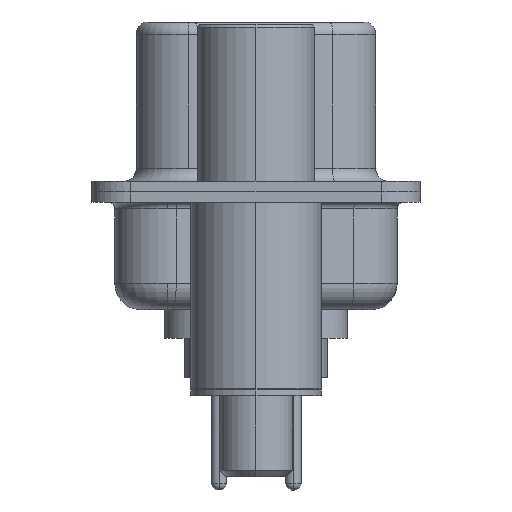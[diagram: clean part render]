
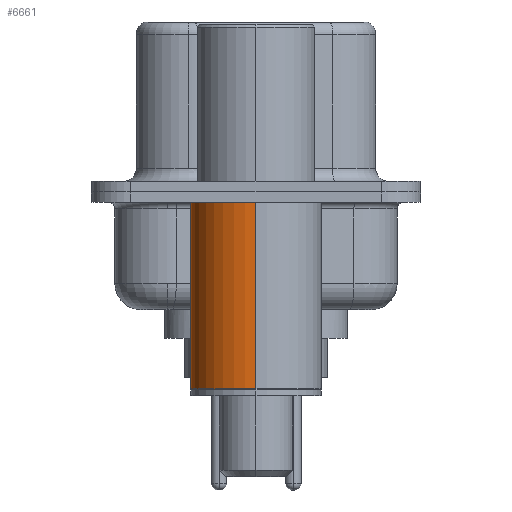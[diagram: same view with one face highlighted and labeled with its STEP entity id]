
A CAD part, left-side view. The second image highlights one B-rep face of the part: STEP entity #6661.
In plain terms, the highlighted cylindrical face has radius 2.5 mm (diameter 5 mm), a partial arc.
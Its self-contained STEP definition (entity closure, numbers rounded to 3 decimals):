
#350 = DIRECTION ( 'NONE',  ( 1., 0., 0. ) ) ;
#1232 = VERTEX_POINT ( 'NONE', #16352 ) ;
#1234 = VERTEX_POINT ( 'NONE', #18870 ) ;
#1271 = DIRECTION ( 'NONE',  ( 1., 0., 0. ) ) ;
#1822 = ORIENTED_EDGE ( 'NONE', *, *, #8953, .T. ) ;
#3179 = AXIS2_PLACEMENT_3D ( 'NONE', #19031, #9683, #350 ) ;
#3250 = CARTESIAN_POINT ( 'NONE',  ( 2.5, 0., -7.525 ) ) ;
#3787 = EDGE_CURVE ( 'NONE', #10739, #1232, #9928, .T. ) ;
#4009 = VECTOR ( 'NONE', #15874, 1000. ) ;
#4331 = DIRECTION ( 'NONE',  ( 1., 0., 0. ) ) ;
#5615 = AXIS2_PLACEMENT_3D ( 'NONE', #13617, #13555, #4331 ) ;
#6210 = ORIENTED_EDGE ( 'NONE', *, *, #3787, .F. ) ;
#6661 = ADVANCED_FACE ( 'NONE', ( #18788 ), #18314, .T. ) ;
#7022 = CIRCLE ( 'NONE', #9948, 2.5 ) ;
#7495 = VECTOR ( 'NONE', #8702, 1000. ) ;
#8129 = LINE ( 'NONE', #12719, #4009 ) ;
#8702 = DIRECTION ( 'NONE',  ( 0., 0., 1. ) ) ;
#8953 = EDGE_CURVE ( 'NONE', #10739, #1234, #13156, .T. ) ;
#9252 = VERTEX_POINT ( 'NONE', #19794 ) ;
#9683 = DIRECTION ( 'NONE',  ( 0., 0., 1. ) ) ;
#9928 = LINE ( 'NONE', #19090, #7495 ) ;
#9948 = AXIS2_PLACEMENT_3D ( 'NONE', #19936, #10584, #1271 ) ;
#10119 = EDGE_CURVE ( 'NONE', #1232, #9252, #7022, .T. ) ;
#10584 = DIRECTION ( 'NONE',  ( 0., 0., 1. ) ) ;
#10739 = VERTEX_POINT ( 'NONE', #3250 ) ;
#12719 = CARTESIAN_POINT ( 'NONE',  ( -2.5, 0., 0.581 ) ) ;
#13156 = CIRCLE ( 'NONE', #3179, 2.5 ) ;
#13549 = ORIENTED_EDGE ( 'NONE', *, *, #10119, .F. ) ;
#13555 = DIRECTION ( 'NONE',  ( 0., 0., 1. ) ) ;
#13617 = CARTESIAN_POINT ( 'NONE',  ( 0., 0., 0.581 ) ) ;
#14818 = ORIENTED_EDGE ( 'NONE', *, *, #16554, .T. ) ;
#15874 = DIRECTION ( 'NONE',  ( 0., 0., 1. ) ) ;
#16143 = EDGE_LOOP ( 'NONE', ( #1822, #14818, #13549, #6210 ) ) ;
#16352 = CARTESIAN_POINT ( 'NONE',  ( 2.5, 0., -0.4 ) ) ;
#16554 = EDGE_CURVE ( 'NONE', #1234, #9252, #8129, .T. ) ;
#18314 = CYLINDRICAL_SURFACE ( 'NONE', #5615, 2.5 ) ;
#18788 = FACE_OUTER_BOUND ( 'NONE', #16143, .T. ) ;
#18870 = CARTESIAN_POINT ( 'NONE',  ( -2.5, 0., -7.525 ) ) ;
#19031 = CARTESIAN_POINT ( 'NONE',  ( 0., 0., -7.525 ) ) ;
#19090 = CARTESIAN_POINT ( 'NONE',  ( 2.5, 0., 0.581 ) ) ;
#19794 = CARTESIAN_POINT ( 'NONE',  ( -2.5, 0., -0.4 ) ) ;
#19936 = CARTESIAN_POINT ( 'NONE',  ( 0., 0., -0.4 ) ) ;
